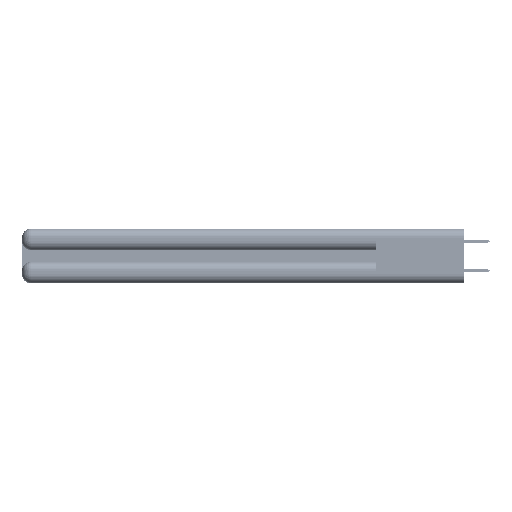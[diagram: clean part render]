
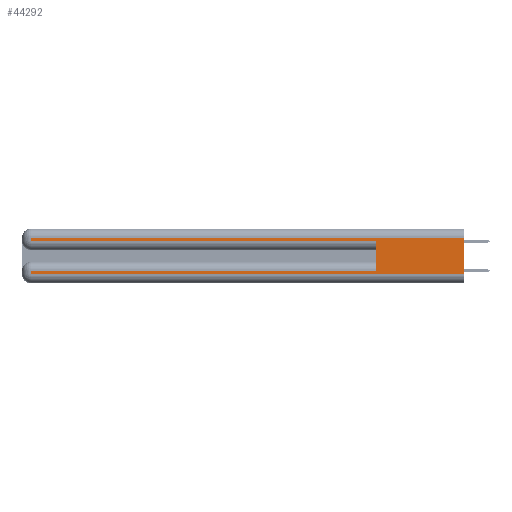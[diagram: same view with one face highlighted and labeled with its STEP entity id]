
A CAD part, left-side view. The second image highlights one B-rep face of the part: STEP entity #44292.
In plain terms, the highlighted planar face has unit normal (-1, 0, 0).
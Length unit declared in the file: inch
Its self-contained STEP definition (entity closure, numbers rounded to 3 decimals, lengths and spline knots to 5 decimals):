
#367 = LINE ( 'NONE', #42532, #11822 ) ;
#639 = LINE ( 'NONE', #41759, #22164 ) ;
#787 = EDGE_CURVE ( 'NONE', #32848, #19007, #31847, .T. ) ;
#1115 = ORIENTED_EDGE ( 'NONE', *, *, #33900, .T. ) ;
#2130 = EDGE_CURVE ( 'NONE', #32848, #33268, #22843, .T. ) ;
#2144 = AXIS2_PLACEMENT_3D ( 'NONE', #54704, #33249, #7391 ) ;
#3080 = PLANE ( 'NONE',  #2144 ) ;
#3435 = FACE_OUTER_BOUND ( 'NONE', #15940, .T. ) ;
#3608 = CARTESIAN_POINT ( 'NONE',  ( 0., 2.94, 0.06 ) ) ;
#4725 = EDGE_CURVE ( 'NONE', #14799, #5433, #23347, .T. ) ;
#5433 = VERTEX_POINT ( 'NONE', #28192 ) ;
#6283 = EDGE_CURVE ( 'NONE', #40249, #5433, #367, .T. ) ;
#7391 = DIRECTION ( 'NONE',  ( 0., 0., -1. ) ) ;
#7821 = LINE ( 'NONE', #49537, #40851 ) ;
#7823 = ORIENTED_EDGE ( 'NONE', *, *, #11716, .T. ) ;
#11039 = CARTESIAN_POINT ( 'NONE',  ( 0., 0., 0.37 ) ) ;
#11716 = EDGE_CURVE ( 'NONE', #45991, #33268, #45193, .T. ) ;
#11822 = VECTOR ( 'NONE', #47050, 39.37008 ) ;
#12135 = VECTOR ( 'NONE', #47749, 39.37008 ) ;
#14648 = CARTESIAN_POINT ( 'NONE',  ( 0., 2.94, 0.285 ) ) ;
#14799 = VERTEX_POINT ( 'NONE', #14648 ) ;
#15094 = CARTESIAN_POINT ( 'NONE',  ( 0., 0., 0.31 ) ) ;
#15927 = CARTESIAN_POINT ( 'NONE',  ( 0., 0., 0.085 ) ) ;
#15940 = EDGE_LOOP ( 'NONE', ( #27510, #35193, #45051, #34411, #41796, #1115, #17775, #7823 ) ) ;
#16602 = LINE ( 'NONE', #15927, #26679 ) ;
#17775 = ORIENTED_EDGE ( 'NONE', *, *, #18824, .T. ) ;
#18324 = CARTESIAN_POINT ( 'NONE',  ( 0., 0.6, 0.085 ) ) ;
#18824 = EDGE_CURVE ( 'NONE', #41107, #45991, #639, .T. ) ;
#19007 = VERTEX_POINT ( 'NONE', #34357 ) ;
#19380 = DIRECTION ( 'NONE',  ( 0., 0., -1. ) ) ;
#19497 = DIRECTION ( 'NONE',  ( 0., 0., -1. ) ) ;
#20305 = VECTOR ( 'NONE', #36648, 39.37008 ) ;
#21989 = VECTOR ( 'NONE', #26916, 39.37008 ) ;
#22164 = VECTOR ( 'NONE', #54778, 39.37008 ) ;
#22614 = CARTESIAN_POINT ( 'NONE',  ( 0., 0., 0.31 ) ) ;
#22843 = LINE ( 'NONE', #11039, #34405 ) ;
#23347 = LINE ( 'NONE', #48416, #21989 ) ;
#26243 = CARTESIAN_POINT ( 'NONE',  ( 0., 0., 0.06 ) ) ;
#26679 = VECTOR ( 'NONE', #54799, 39.37008 ) ;
#26916 = DIRECTION ( 'NONE',  ( 0., -1., 0. ) ) ;
#27510 = ORIENTED_EDGE ( 'NONE', *, *, #2130, .F. ) ;
#28192 = CARTESIAN_POINT ( 'NONE',  ( 0., 0.6, 0.285 ) ) ;
#29405 = CARTESIAN_POINT ( 'NONE',  ( 0., 0., 0.06 ) ) ;
#31847 = LINE ( 'NONE', #15094, #20305 ) ;
#32848 = VERTEX_POINT ( 'NONE', #22614 ) ;
#33249 = DIRECTION ( 'NONE',  ( 1., 0., 0. ) ) ;
#33268 = VERTEX_POINT ( 'NONE', #29405 ) ;
#33900 = EDGE_CURVE ( 'NONE', #40249, #41107, #16602, .T. ) ;
#34357 = CARTESIAN_POINT ( 'NONE',  ( 0., 2.94, 0.31 ) ) ;
#34405 = VECTOR ( 'NONE', #19497, 39.37008 ) ;
#34411 = ORIENTED_EDGE ( 'NONE', *, *, #4725, .T. ) ;
#35193 = ORIENTED_EDGE ( 'NONE', *, *, #787, .T. ) ;
#36648 = DIRECTION ( 'NONE',  ( 0., 1., 0. ) ) ;
#40249 = VERTEX_POINT ( 'NONE', #18324 ) ;
#40851 = VECTOR ( 'NONE', #19380, 39.37008 ) ;
#40977 = EDGE_CURVE ( 'NONE', #19007, #14799, #7821, .T. ) ;
#41107 = VERTEX_POINT ( 'NONE', #50281 ) ;
#41759 = CARTESIAN_POINT ( 'NONE',  ( 0., 2.94, 0.37 ) ) ;
#41796 = ORIENTED_EDGE ( 'NONE', *, *, #6283, .F. ) ;
#42532 = CARTESIAN_POINT ( 'NONE',  ( 0., 0.6, 0.145 ) ) ;
#44292 = ADVANCED_FACE ( 'NONE', ( #3435 ), #3080, .F. ) ;
#45051 = ORIENTED_EDGE ( 'NONE', *, *, #40977, .T. ) ;
#45193 = LINE ( 'NONE', #26243, #12135 ) ;
#45991 = VERTEX_POINT ( 'NONE', #3608 ) ;
#47050 = DIRECTION ( 'NONE',  ( 0., 0., 1. ) ) ;
#47749 = DIRECTION ( 'NONE',  ( 0., -1., 0. ) ) ;
#48416 = CARTESIAN_POINT ( 'NONE',  ( 0., 0., 0.285 ) ) ;
#49537 = CARTESIAN_POINT ( 'NONE',  ( 0., 2.94, 0.37 ) ) ;
#50281 = CARTESIAN_POINT ( 'NONE',  ( 0., 2.94, 0.085 ) ) ;
#54704 = CARTESIAN_POINT ( 'NONE',  ( 0., 0., 0.37 ) ) ;
#54778 = DIRECTION ( 'NONE',  ( 0., 0., -1. ) ) ;
#54799 = DIRECTION ( 'NONE',  ( 0., 1., 0. ) ) ;
